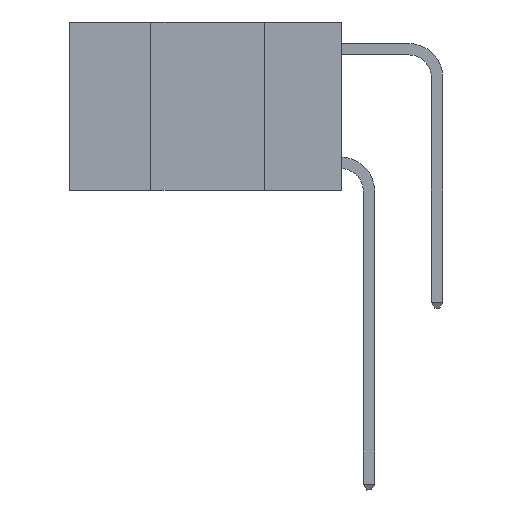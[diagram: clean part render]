
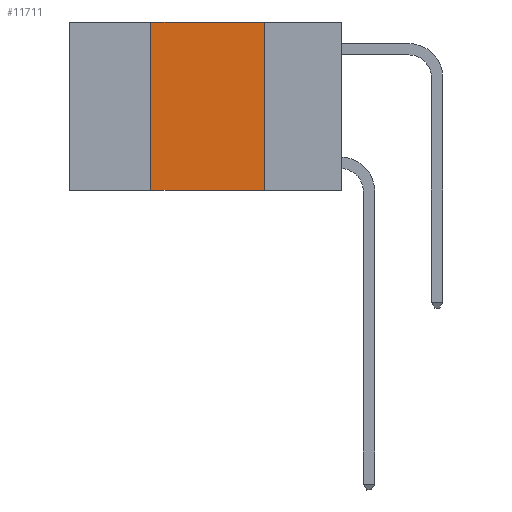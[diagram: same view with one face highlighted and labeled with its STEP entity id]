
A CAD part, left-side view. The second image highlights one B-rep face of the part: STEP entity #11711.
In plain terms, the highlighted planar face has unit normal (-1, 0, 0).
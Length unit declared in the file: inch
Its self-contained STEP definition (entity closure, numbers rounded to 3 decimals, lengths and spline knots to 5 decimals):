
#464 = EDGE_CURVE ( 'NONE', #9102, #1542, #8909, .T. ) ;
#1307 = CARTESIAN_POINT ( 'NONE',  ( 0., 0.42, -0.37 ) ) ;
#1542 = VERTEX_POINT ( 'NONE', #3345 ) ;
#3122 = EDGE_CURVE ( 'NONE', #1542, #10011, #3973, .T. ) ;
#3345 = CARTESIAN_POINT ( 'NONE',  ( 0., 0.17, 0. ) ) ;
#3435 = VERTEX_POINT ( 'NONE', #1307 ) ;
#3553 = DIRECTION ( 'NONE',  ( 1., 0., 0. ) ) ;
#3973 = LINE ( 'NONE', #10647, #8862 ) ;
#4068 = ORIENTED_EDGE ( 'NONE', *, *, #10054, .F. ) ;
#4194 = LINE ( 'NONE', #10264, #9400 ) ;
#4306 = CARTESIAN_POINT ( 'NONE',  ( 0., 0.6, -0.37 ) ) ;
#4309 = ORIENTED_EDGE ( 'NONE', *, *, #464, .F. ) ;
#4537 = VECTOR ( 'NONE', #6350, 39.37008 ) ;
#4895 = CARTESIAN_POINT ( 'NONE',  ( 0., 0.17, -0.37 ) ) ;
#5924 = DIRECTION ( 'NONE',  ( 0., 0., 1. ) ) ;
#6253 = CARTESIAN_POINT ( 'NONE',  ( 0., 0.42, 0. ) ) ;
#6350 = DIRECTION ( 'NONE',  ( 0., -1., 0. ) ) ;
#6903 = ORIENTED_EDGE ( 'NONE', *, *, #3122, .F. ) ;
#7135 = LINE ( 'NONE', #4306, #4537 ) ;
#7457 = PLANE ( 'NONE',  #10986 ) ;
#7976 = FACE_OUTER_BOUND ( 'NONE', #8008, .T. ) ;
#8008 = EDGE_LOOP ( 'NONE', ( #6903, #4309, #4068, #11012 ) ) ;
#8862 = VECTOR ( 'NONE', #11608, 39.37008 ) ;
#8909 = LINE ( 'NONE', #9321, #11473 ) ;
#9102 = VERTEX_POINT ( 'NONE', #6253 ) ;
#9156 = EDGE_CURVE ( 'NONE', #3435, #10011, #7135, .T. ) ;
#9274 = DIRECTION ( 'NONE',  ( 0., -1., 0. ) ) ;
#9321 = CARTESIAN_POINT ( 'NONE',  ( 0., 0.6, 0. ) ) ;
#9400 = VECTOR ( 'NONE', #5924, 39.37008 ) ;
#9414 = CARTESIAN_POINT ( 'NONE',  ( 0., 0.6, 0. ) ) ;
#10011 = VERTEX_POINT ( 'NONE', #4895 ) ;
#10054 = EDGE_CURVE ( 'NONE', #3435, #9102, #4194, .T. ) ;
#10264 = CARTESIAN_POINT ( 'NONE',  ( 0., 0.42, 0. ) ) ;
#10386 = DIRECTION ( 'NONE',  ( 0., 0., -1. ) ) ;
#10647 = CARTESIAN_POINT ( 'NONE',  ( 0., 0.17, 0. ) ) ;
#10986 = AXIS2_PLACEMENT_3D ( 'NONE', #9414, #3553, #10386 ) ;
#11012 = ORIENTED_EDGE ( 'NONE', *, *, #9156, .T. ) ;
#11473 = VECTOR ( 'NONE', #9274, 39.37008 ) ;
#11608 = DIRECTION ( 'NONE',  ( 0., 0., -1. ) ) ;
#11711 = ADVANCED_FACE ( 'NONE', ( #7976 ), #7457, .F. ) ;
